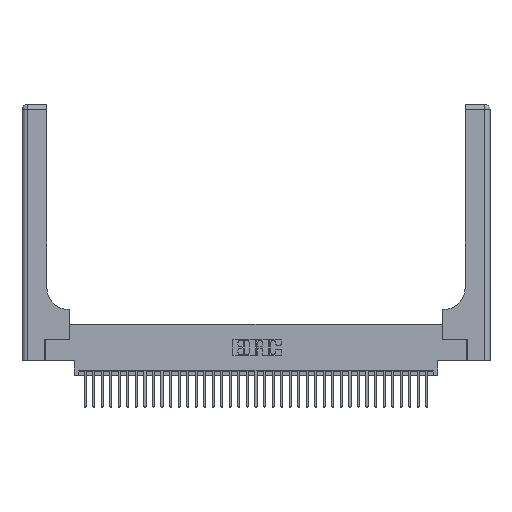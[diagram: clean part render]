
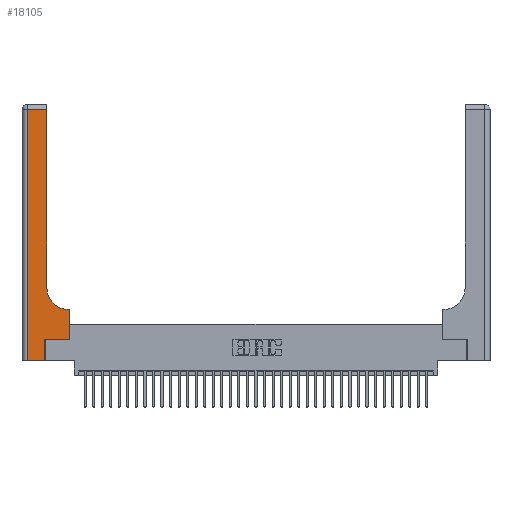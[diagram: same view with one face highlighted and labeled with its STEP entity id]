
A CAD part, top view. The second image highlights one B-rep face of the part: STEP entity #18105.
In plain terms, the highlighted planar face has unit normal (0, 0, 1).
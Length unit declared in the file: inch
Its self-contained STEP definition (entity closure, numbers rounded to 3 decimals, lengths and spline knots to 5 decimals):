
#90 = CARTESIAN_POINT ( 'NONE',  ( 0.5415, 0.6, 0.37 ) ) ;
#176 = DIRECTION ( 'NONE',  ( 0., 1., 0. ) ) ;
#395 = ORIENTED_EDGE ( 'NONE', *, *, #2660, .T. ) ;
#654 = LINE ( 'NONE', #31141, #20235 ) ;
#2660 = EDGE_CURVE ( 'NONE', #21183, #3350, #37373, .T. ) ;
#3253 = VERTEX_POINT ( 'NONE', #29405 ) ;
#3350 = VERTEX_POINT ( 'NONE', #27214 ) ;
#3633 = ORIENTED_EDGE ( 'NONE', *, *, #7423, .T. ) ;
#3723 = CARTESIAN_POINT ( 'NONE',  ( 0.06, 2.94, 0.37 ) ) ;
#4941 = ORIENTED_EDGE ( 'NONE', *, *, #7687, .T. ) ;
#5101 = CARTESIAN_POINT ( 'NONE',  ( 0.269, 0.25, 0.37 ) ) ;
#7374 = ORIENTED_EDGE ( 'NONE', *, *, #12918, .T. ) ;
#7423 = EDGE_CURVE ( 'NONE', #21500, #31357, #11181, .T. ) ;
#7687 = EDGE_CURVE ( 'NONE', #20720, #21500, #20754, .T. ) ;
#7756 = CARTESIAN_POINT ( 'NONE',  ( 0.06, 0., 0.37 ) ) ;
#8113 = DIRECTION ( 'NONE',  ( 0., 0., -1. ) ) ;
#8203 = VERTEX_POINT ( 'NONE', #3723 ) ;
#8716 = EDGE_CURVE ( 'NONE', #8203, #20720, #654, .T. ) ;
#9809 = EDGE_CURVE ( 'NONE', #24908, #8203, #27933, .T. ) ;
#10334 = CARTESIAN_POINT ( 'NONE',  ( 0.269, 0.25, 0.37 ) ) ;
#10927 = AXIS2_PLACEMENT_3D ( 'NONE', #12519, #8113, #19726 ) ;
#11090 = LINE ( 'NONE', #23305, #22977 ) ;
#11181 = LINE ( 'NONE', #19279, #18065 ) ;
#11749 = DIRECTION ( 'NONE',  ( 1., 0., 0. ) ) ;
#12519 = CARTESIAN_POINT ( 'NONE',  ( 0., 3., 0.37 ) ) ;
#12918 = EDGE_CURVE ( 'NONE', #30392, #3253, #26603, .T. ) ;
#13300 = DIRECTION ( 'NONE',  ( 1., 0., 0. ) ) ;
#13915 = VECTOR ( 'NONE', #11749, 39.37008 ) ;
#14352 = CARTESIAN_POINT ( 'NONE',  ( 0.2915, 2.94, 0.37 ) ) ;
#14999 = LINE ( 'NONE', #5101, #18179 ) ;
#15425 = ORIENTED_EDGE ( 'NONE', *, *, #21378, .T. ) ;
#15635 = EDGE_CURVE ( 'NONE', #31357, #21183, #14999, .T. ) ;
#16551 = VECTOR ( 'NONE', #176, 39.37008 ) ;
#16710 = DIRECTION ( 'NONE',  ( 1., 0., 0. ) ) ;
#17322 = DIRECTION ( 'NONE',  ( -1., 0., 0. ) ) ;
#17491 = VECTOR ( 'NONE', #17540, 39.37008 ) ;
#17540 = DIRECTION ( 'NONE',  ( -1., 0., 0. ) ) ;
#18065 = VECTOR ( 'NONE', #36657, 39.37008 ) ;
#18105 = ADVANCED_FACE ( 'NONE', ( #34941 ), #33342, .F. ) ;
#18179 = VECTOR ( 'NONE', #13300, 39.37008 ) ;
#19209 = ORIENTED_EDGE ( 'NONE', *, *, #9809, .T. ) ;
#19279 = CARTESIAN_POINT ( 'NONE',  ( 0.269, 0., 0.37 ) ) ;
#19430 = ORIENTED_EDGE ( 'NONE', *, *, #15635, .T. ) ;
#19491 = CARTESIAN_POINT ( 'NONE',  ( 0.5415, 0.85, 0.37 ) ) ;
#19726 = DIRECTION ( 'NONE',  ( -1., 0., 0. ) ) ;
#20235 = VECTOR ( 'NONE', #33685, 39.37008 ) ;
#20720 = VERTEX_POINT ( 'NONE', #7756 ) ;
#20754 = LINE ( 'NONE', #37529, #13915 ) ;
#21183 = VERTEX_POINT ( 'NONE', #27356 ) ;
#21378 = EDGE_CURVE ( 'NONE', #3350, #30392, #11090, .T. ) ;
#21500 = VERTEX_POINT ( 'NONE', #29618 ) ;
#21985 = EDGE_CURVE ( 'NONE', #3253, #24908, #22022, .T. ) ;
#22022 = LINE ( 'NONE', #23006, #16551 ) ;
#22977 = VECTOR ( 'NONE', #17322, 39.37008 ) ;
#23006 = CARTESIAN_POINT ( 'NONE',  ( 0.2915, 3., 0.37 ) ) ;
#23239 = EDGE_LOOP ( 'NONE', ( #28875, #19209, #23471, #4941, #3633, #19430, #395, #15425, #7374 ) ) ;
#23305 = CARTESIAN_POINT ( 'NONE',  ( 0.2915, 0.6, 0.37 ) ) ;
#23471 = ORIENTED_EDGE ( 'NONE', *, *, #8716, .T. ) ;
#24548 = CARTESIAN_POINT ( 'NONE',  ( 0.5585, 0.25, 0.37 ) ) ;
#24681 = DIRECTION ( 'NONE',  ( 0., 1., 0. ) ) ;
#24908 = VERTEX_POINT ( 'NONE', #14352 ) ;
#25108 = DIRECTION ( 'NONE',  ( 0., 0., -1. ) ) ;
#25306 = AXIS2_PLACEMENT_3D ( 'NONE', #19491, #25108, #16710 ) ;
#26603 = CIRCLE ( 'NONE', #25306, 0.25 ) ;
#27214 = CARTESIAN_POINT ( 'NONE',  ( 0.5585, 0.6, 0.37 ) ) ;
#27356 = CARTESIAN_POINT ( 'NONE',  ( 0.5585, 0.25, 0.37 ) ) ;
#27933 = LINE ( 'NONE', #32489, #17491 ) ;
#28875 = ORIENTED_EDGE ( 'NONE', *, *, #21985, .T. ) ;
#29183 = VECTOR ( 'NONE', #24681, 39.37008 ) ;
#29405 = CARTESIAN_POINT ( 'NONE',  ( 0.2915, 0.85, 0.37 ) ) ;
#29618 = CARTESIAN_POINT ( 'NONE',  ( 0.269, 0., 0.37 ) ) ;
#30392 = VERTEX_POINT ( 'NONE', #90 ) ;
#31141 = CARTESIAN_POINT ( 'NONE',  ( 0.06, 3., 0.37 ) ) ;
#31357 = VERTEX_POINT ( 'NONE', #10334 ) ;
#32489 = CARTESIAN_POINT ( 'NONE',  ( 0., 2.94, 0.37 ) ) ;
#33342 = PLANE ( 'NONE',  #10927 ) ;
#33685 = DIRECTION ( 'NONE',  ( 0., -1., 0. ) ) ;
#34941 = FACE_OUTER_BOUND ( 'NONE', #23239, .T. ) ;
#36657 = DIRECTION ( 'NONE',  ( 0., 1., 0. ) ) ;
#37373 = LINE ( 'NONE', #24548, #29183 ) ;
#37529 = CARTESIAN_POINT ( 'NONE',  ( 0., 0., 0.37 ) ) ;
